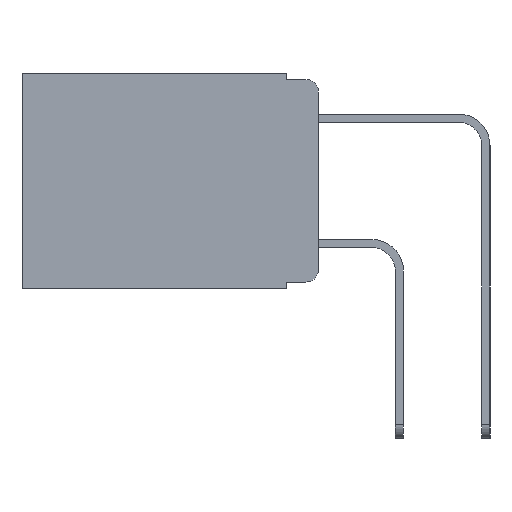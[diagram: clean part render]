
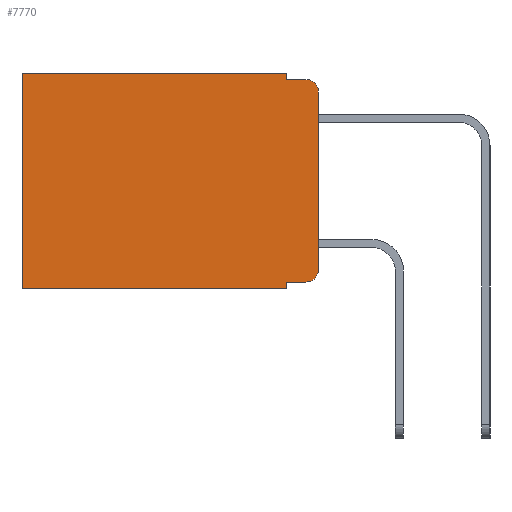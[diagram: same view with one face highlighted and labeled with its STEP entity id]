
A CAD part, left-side view. The second image highlights one B-rep face of the part: STEP entity #7770.
In plain terms, the highlighted planar face has unit normal (-1, 0, 0).
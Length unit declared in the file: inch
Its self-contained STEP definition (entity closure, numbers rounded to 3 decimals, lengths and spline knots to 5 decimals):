
#21 = AXIS2_PLACEMENT_3D ( 'NONE', #19227, #10647, #1035 ) ;
#543 = EDGE_CURVE ( 'NONE', #9584, #10422, #6410, .T. ) ;
#689 = CARTESIAN_POINT ( 'NONE',  ( 0.298, 0.051, -0.333 ) ) ;
#1035 = DIRECTION ( 'NONE',  ( 0., 0., -1. ) ) ;
#1272 = CARTESIAN_POINT ( 'NONE',  ( 0.298, 0.051, -0.01 ) ) ;
#1484 = CARTESIAN_POINT ( 'NONE',  ( 0.298, 0., 0. ) ) ;
#1579 = DIRECTION ( 'NONE',  ( 0., 0., -1. ) ) ;
#1657 = EDGE_CURVE ( 'NONE', #3799, #12128, #9566, .T. ) ;
#1709 = LINE ( 'NONE', #9351, #16999 ) ;
#1948 = ORIENTED_EDGE ( 'NONE', *, *, #1657, .T. ) ;
#2004 = CARTESIAN_POINT ( 'NONE',  ( 0.298, 0.051, -0.333 ) ) ;
#2229 = CARTESIAN_POINT ( 'NONE',  ( 0.298, 0., -0.313 ) ) ;
#3023 = EDGE_CURVE ( 'NONE', #10422, #13447, #12852, .T. ) ;
#3799 = VERTEX_POINT ( 'NONE', #14793 ) ;
#4083 = EDGE_CURVE ( 'NONE', #12069, #14294, #1709, .T. ) ;
#4097 = ORIENTED_EDGE ( 'NONE', *, *, #18860, .T. ) ;
#4153 = FACE_OUTER_BOUND ( 'NONE', #8949, .T. ) ;
#4227 = CARTESIAN_POINT ( 'NONE',  ( 0.298, 0., 0. ) ) ;
#4545 = CARTESIAN_POINT ( 'NONE',  ( 0.298, 0.473, -0.343 ) ) ;
#4636 = VECTOR ( 'NONE', #8922, 39.37008 ) ;
#5728 = CARTESIAN_POINT ( 'NONE',  ( 0.298, 0., -0.03 ) ) ;
#6133 = LINE ( 'NONE', #6161, #9813 ) ;
#6161 = CARTESIAN_POINT ( 'NONE',  ( 0.298, 0.051, 0. ) ) ;
#6237 = EDGE_CURVE ( 'NONE', #14066, #12128, #19164, .T. ) ;
#6267 = ORIENTED_EDGE ( 'NONE', *, *, #13265, .F. ) ;
#6410 = LINE ( 'NONE', #4227, #17785 ) ;
#6412 = CARTESIAN_POINT ( 'NONE',  ( 0.298, 0., 0. ) ) ;
#6755 = ORIENTED_EDGE ( 'NONE', *, *, #4083, .F. ) ;
#7272 = DIRECTION ( 'NONE',  ( 0., -1., 0. ) ) ;
#7414 = VERTEX_POINT ( 'NONE', #11805 ) ;
#7770 = ADVANCED_FACE ( 'NONE', ( #4153 ), #18256, .F. ) ;
#7778 = DIRECTION ( 'NONE',  ( 0., 0., -1. ) ) ;
#8092 = DIRECTION ( 'NONE',  ( 0., 0., -1. ) ) ;
#8922 = DIRECTION ( 'NONE',  ( 0., 0., -1. ) ) ;
#8949 = EDGE_LOOP ( 'NONE', ( #12799, #4097, #15881, #11880, #14786, #18527, #6267, #6755, #15856, #1948 ) ) ;
#9300 = DIRECTION ( 'NONE',  ( 0., -1., 0. ) ) ;
#9351 = CARTESIAN_POINT ( 'NONE',  ( 0.298, 0.051, 0. ) ) ;
#9541 = DIRECTION ( 'NONE',  ( -1., 0., 0. ) ) ;
#9566 = CIRCLE ( 'NONE', #21, 0.02 ) ;
#9584 = VERTEX_POINT ( 'NONE', #15092 ) ;
#9789 = VECTOR ( 'NONE', #9300, 39.37008 ) ;
#9813 = VECTOR ( 'NONE', #7778, 39.37008 ) ;
#9972 = VERTEX_POINT ( 'NONE', #18246 ) ;
#10056 = CARTESIAN_POINT ( 'NONE',  ( 0.298, 0., -0.343 ) ) ;
#10088 = DIRECTION ( 'NONE',  ( 0., 1., 0. ) ) ;
#10422 = VERTEX_POINT ( 'NONE', #15450 ) ;
#10647 = DIRECTION ( 'NONE',  ( -1., 0., 0. ) ) ;
#11129 = DIRECTION ( 'NONE',  ( 1., 0., 0. ) ) ;
#11621 = VECTOR ( 'NONE', #8092, 39.37008 ) ;
#11684 = DIRECTION ( 'NONE',  ( 0., 1., 0. ) ) ;
#11805 = CARTESIAN_POINT ( 'NONE',  ( 0.298, 0.051, -0.01 ) ) ;
#11880 = ORIENTED_EDGE ( 'NONE', *, *, #12867, .F. ) ;
#12069 = VERTEX_POINT ( 'NONE', #2004 ) ;
#12128 = VERTEX_POINT ( 'NONE', #2229 ) ;
#12273 = AXIS2_PLACEMENT_3D ( 'NONE', #18222, #9541, #19648 ) ;
#12799 = ORIENTED_EDGE ( 'NONE', *, *, #6237, .F. ) ;
#12845 = VECTOR ( 'NONE', #7272, 39.37008 ) ;
#12852 = LINE ( 'NONE', #14874, #4636 ) ;
#12867 = EDGE_CURVE ( 'NONE', #9584, #7414, #6133, .T. ) ;
#13097 = AXIS2_PLACEMENT_3D ( 'NONE', #6412, #11129, #1579 ) ;
#13265 = EDGE_CURVE ( 'NONE', #14294, #13447, #19278, .T. ) ;
#13447 = VERTEX_POINT ( 'NONE', #4545 ) ;
#13727 = CARTESIAN_POINT ( 'NONE',  ( 0.298, 0.051, -0.343 ) ) ;
#14066 = VERTEX_POINT ( 'NONE', #5728 ) ;
#14294 = VERTEX_POINT ( 'NONE', #13727 ) ;
#14786 = ORIENTED_EDGE ( 'NONE', *, *, #543, .T. ) ;
#14793 = CARTESIAN_POINT ( 'NONE',  ( 0.298, 0.02, -0.333 ) ) ;
#14874 = CARTESIAN_POINT ( 'NONE',  ( 0.298, 0.473, 0. ) ) ;
#15092 = CARTESIAN_POINT ( 'NONE',  ( 0.298, 0.051, 0. ) ) ;
#15272 = DIRECTION ( 'NONE',  ( 0., 0., -1. ) ) ;
#15450 = CARTESIAN_POINT ( 'NONE',  ( 0.298, 0.473, 0. ) ) ;
#15529 = VECTOR ( 'NONE', #11684, 39.37008 ) ;
#15856 = ORIENTED_EDGE ( 'NONE', *, *, #19294, .T. ) ;
#15881 = ORIENTED_EDGE ( 'NONE', *, *, #18208, .F. ) ;
#16143 = CIRCLE ( 'NONE', #12273, 0.02 ) ;
#16566 = LINE ( 'NONE', #689, #12845 ) ;
#16999 = VECTOR ( 'NONE', #15272, 39.37008 ) ;
#17785 = VECTOR ( 'NONE', #10088, 39.37008 ) ;
#18208 = EDGE_CURVE ( 'NONE', #7414, #9972, #18391, .T. ) ;
#18222 = CARTESIAN_POINT ( 'NONE',  ( 0.298, 0.02, -0.03 ) ) ;
#18246 = CARTESIAN_POINT ( 'NONE',  ( 0.298, 0.02, -0.01 ) ) ;
#18256 = PLANE ( 'NONE',  #13097 ) ;
#18391 = LINE ( 'NONE', #1272, #9789 ) ;
#18527 = ORIENTED_EDGE ( 'NONE', *, *, #3023, .T. ) ;
#18860 = EDGE_CURVE ( 'NONE', #14066, #9972, #16143, .T. ) ;
#19164 = LINE ( 'NONE', #1484, #11621 ) ;
#19227 = CARTESIAN_POINT ( 'NONE',  ( 0.298, 0.02, -0.313 ) ) ;
#19278 = LINE ( 'NONE', #10056, #15529 ) ;
#19294 = EDGE_CURVE ( 'NONE', #12069, #3799, #16566, .T. ) ;
#19648 = DIRECTION ( 'NONE',  ( 0., 0., -1. ) ) ;
